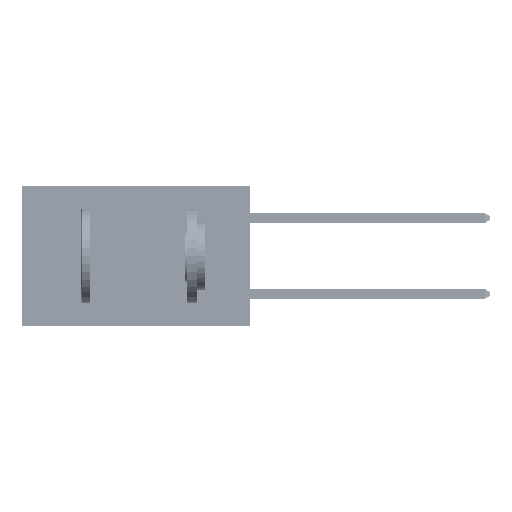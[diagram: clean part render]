
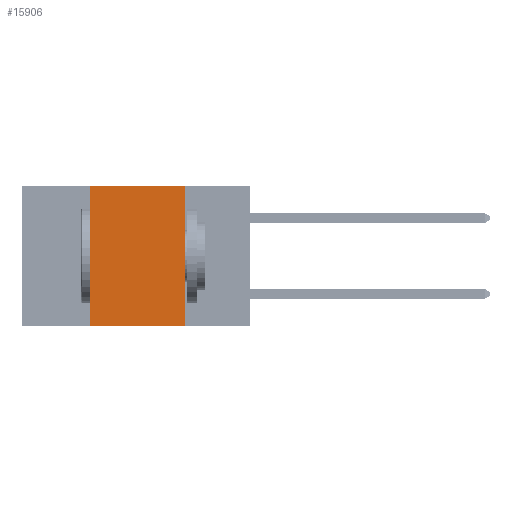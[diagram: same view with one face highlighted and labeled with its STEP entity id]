
A CAD part, left-side view. The second image highlights one B-rep face of the part: STEP entity #15906.
In plain terms, the highlighted planar face has unit normal (-1, 0, 0).
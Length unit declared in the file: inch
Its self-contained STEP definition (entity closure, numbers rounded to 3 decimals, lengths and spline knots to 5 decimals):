
#330 = CARTESIAN_POINT ( 'NONE',  ( 0., 0.17, -0.37 ) ) ;
#2119 = AXIS2_PLACEMENT_3D ( 'NONE', #36238, #3901, #11920 ) ;
#3901 = DIRECTION ( 'NONE',  ( 1., 0., 0. ) ) ;
#4986 = VERTEX_POINT ( 'NONE', #13582 ) ;
#5152 = EDGE_CURVE ( 'NONE', #49417, #4986, #6915, .T. ) ;
#6308 = ORIENTED_EDGE ( 'NONE', *, *, #51869, .T. ) ;
#6915 = LINE ( 'NONE', #31655, #34277 ) ;
#8478 = EDGE_LOOP ( 'NONE', ( #41218, #38378, #10182, #6308 ) ) ;
#10182 = ORIENTED_EDGE ( 'NONE', *, *, #5152, .F. ) ;
#11920 = DIRECTION ( 'NONE',  ( 0., 0., -1. ) ) ;
#13582 = CARTESIAN_POINT ( 'NONE',  ( 0., 0.42, 0. ) ) ;
#15906 = ADVANCED_FACE ( 'NONE', ( #29413 ), #35897, .F. ) ;
#16702 = VECTOR ( 'NONE', #21539, 39.37008 ) ;
#17662 = VECTOR ( 'NONE', #18818, 39.37008 ) ;
#18818 = DIRECTION ( 'NONE',  ( 0., -1., 0. ) ) ;
#21539 = DIRECTION ( 'NONE',  ( 0., 0., -1. ) ) ;
#23062 = EDGE_CURVE ( 'NONE', #4986, #41687, #47972, .T. ) ;
#24165 = CARTESIAN_POINT ( 'NONE',  ( 0., 0.6, 0. ) ) ;
#27180 = CARTESIAN_POINT ( 'NONE',  ( 0., 0.6, -0.37 ) ) ;
#28241 = DIRECTION ( 'NONE',  ( 0., -1., 0. ) ) ;
#28760 = LINE ( 'NONE', #30040, #16702 ) ;
#29413 = FACE_OUTER_BOUND ( 'NONE', #8478, .T. ) ;
#30040 = CARTESIAN_POINT ( 'NONE',  ( 0., 0.17, 0. ) ) ;
#31655 = CARTESIAN_POINT ( 'NONE',  ( 0., 0.42, 0. ) ) ;
#34202 = CARTESIAN_POINT ( 'NONE',  ( 0., 0.17, 0. ) ) ;
#34277 = VECTOR ( 'NONE', #40008, 39.37008 ) ;
#34452 = CARTESIAN_POINT ( 'NONE',  ( 0., 0.42, -0.37 ) ) ;
#35897 = PLANE ( 'NONE',  #2119 ) ;
#36238 = CARTESIAN_POINT ( 'NONE',  ( 0., 0.6, 0. ) ) ;
#38378 = ORIENTED_EDGE ( 'NONE', *, *, #23062, .F. ) ;
#39174 = VERTEX_POINT ( 'NONE', #330 ) ;
#40008 = DIRECTION ( 'NONE',  ( 0., 0., 1. ) ) ;
#41218 = ORIENTED_EDGE ( 'NONE', *, *, #45570, .F. ) ;
#41687 = VERTEX_POINT ( 'NONE', #34202 ) ;
#42261 = VECTOR ( 'NONE', #28241, 39.37008 ) ;
#43125 = LINE ( 'NONE', #27180, #17662 ) ;
#45570 = EDGE_CURVE ( 'NONE', #41687, #39174, #28760, .T. ) ;
#47972 = LINE ( 'NONE', #24165, #42261 ) ;
#49417 = VERTEX_POINT ( 'NONE', #34452 ) ;
#51869 = EDGE_CURVE ( 'NONE', #49417, #39174, #43125, .T. ) ;
